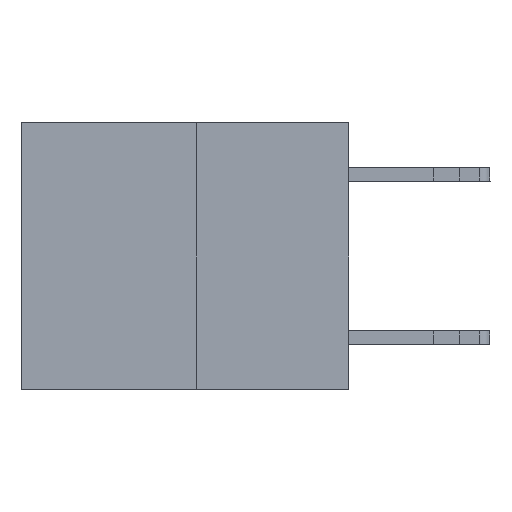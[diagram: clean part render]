
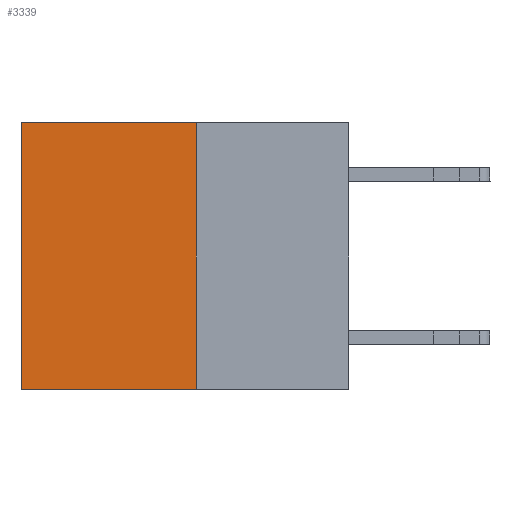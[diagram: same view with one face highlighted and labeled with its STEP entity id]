
A CAD part, left-side view. The second image highlights one B-rep face of the part: STEP entity #3339.
In plain terms, the highlighted planar face has unit normal (-1, 0, 0).
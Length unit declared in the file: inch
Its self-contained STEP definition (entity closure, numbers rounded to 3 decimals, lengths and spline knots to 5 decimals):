
#360 = ORIENTED_EDGE ( 'NONE', *, *, #21880, .F. ) ;
#799 = DIRECTION ( 'NONE',  ( 0., 1., 0. ) ) ;
#834 = VERTEX_POINT ( 'NONE', #22263 ) ;
#990 = EDGE_LOOP ( 'NONE', ( #11181, #360, #3397, #8753 ) ) ;
#1566 = VECTOR ( 'NONE', #24126, 39.37008 ) ;
#1807 = VECTOR ( 'NONE', #20885, 39.37008 ) ;
#2291 = CARTESIAN_POINT ( 'NONE',  ( 0.3165, 0.28, -0.49 ) ) ;
#2665 = VERTEX_POINT ( 'NONE', #20845 ) ;
#3238 = LINE ( 'NONE', #20670, #18572 ) ;
#3339 = ADVANCED_FACE ( 'NONE', ( #23659 ), #9942, .F. ) ;
#3397 = ORIENTED_EDGE ( 'NONE', *, *, #7048, .F. ) ;
#3776 = VERTEX_POINT ( 'NONE', #22798 ) ;
#4797 = CARTESIAN_POINT ( 'NONE',  ( 0.3165, 0.28, 0. ) ) ;
#6013 = LINE ( 'NONE', #4797, #21122 ) ;
#6937 = LINE ( 'NONE', #17708, #1566 ) ;
#7048 = EDGE_CURVE ( 'NONE', #20458, #834, #17182, .T. ) ;
#7992 = DIRECTION ( 'NONE',  ( 1., 0., 0. ) ) ;
#8753 = ORIENTED_EDGE ( 'NONE', *, *, #15661, .T. ) ;
#9688 = DIRECTION ( 'NONE',  ( 0., 0., -1. ) ) ;
#9942 = PLANE ( 'NONE',  #10983 ) ;
#10497 = CARTESIAN_POINT ( 'NONE',  ( 0.3165, 0.28, 0. ) ) ;
#10983 = AXIS2_PLACEMENT_3D ( 'NONE', #18237, #7992, #9688 ) ;
#11181 = ORIENTED_EDGE ( 'NONE', *, *, #12296, .T. ) ;
#12296 = EDGE_CURVE ( 'NONE', #3776, #2665, #6937, .T. ) ;
#15661 = EDGE_CURVE ( 'NONE', #20458, #3776, #6013, .T. ) ;
#17182 = LINE ( 'NONE', #2291, #1807 ) ;
#17708 = CARTESIAN_POINT ( 'NONE',  ( 0.3165, 0.6, -0.49 ) ) ;
#18237 = CARTESIAN_POINT ( 'NONE',  ( 0.3165, 0.28, -0.49 ) ) ;
#18572 = VECTOR ( 'NONE', #24583, 39.37008 ) ;
#20458 = VERTEX_POINT ( 'NONE', #10497 ) ;
#20670 = CARTESIAN_POINT ( 'NONE',  ( 0.3165, 0.28, -0.49 ) ) ;
#20845 = CARTESIAN_POINT ( 'NONE',  ( 0.3165, 0.6, -0.49 ) ) ;
#20885 = DIRECTION ( 'NONE',  ( 0., 0., -1. ) ) ;
#21122 = VECTOR ( 'NONE', #799, 39.37008 ) ;
#21880 = EDGE_CURVE ( 'NONE', #834, #2665, #3238, .T. ) ;
#22263 = CARTESIAN_POINT ( 'NONE',  ( 0.3165, 0.28, -0.49 ) ) ;
#22798 = CARTESIAN_POINT ( 'NONE',  ( 0.3165, 0.6, 0. ) ) ;
#23659 = FACE_OUTER_BOUND ( 'NONE', #990, .T. ) ;
#24126 = DIRECTION ( 'NONE',  ( 0., 0., -1. ) ) ;
#24583 = DIRECTION ( 'NONE',  ( 0., 1., 0. ) ) ;
